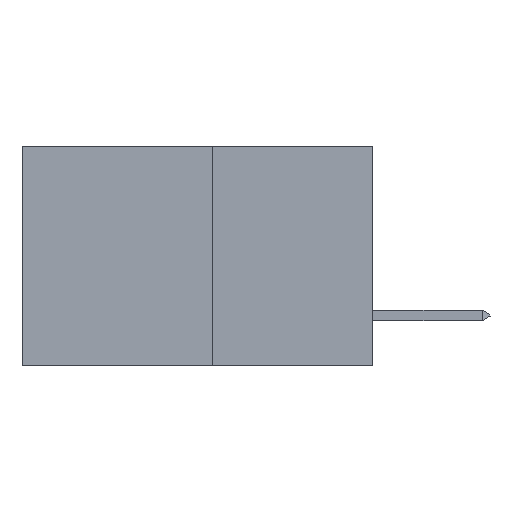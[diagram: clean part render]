
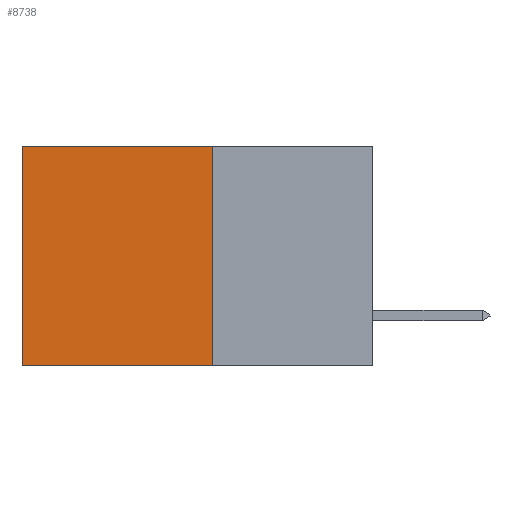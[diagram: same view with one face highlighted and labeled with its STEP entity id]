
A CAD part, left-side view. The second image highlights one B-rep face of the part: STEP entity #8738.
In plain terms, the highlighted planar face has unit normal (-1, 0, 0).
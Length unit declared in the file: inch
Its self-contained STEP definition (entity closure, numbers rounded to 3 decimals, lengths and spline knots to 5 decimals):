
#4 = CARTESIAN_POINT ( 'NONE',  ( 0.277, 0.27, -0.37 ) ) ;
#150 = CARTESIAN_POINT ( 'NONE',  ( 0.277, 0.59, 0. ) ) ;
#162 = EDGE_LOOP ( 'NONE', ( #10276, #10922, #11803, #12343 ) ) ;
#548 = EDGE_CURVE ( 'NONE', #7776, #759, #12877, .T. ) ;
#759 = VERTEX_POINT ( 'NONE', #3535 ) ;
#1396 = VECTOR ( 'NONE', #1722, 39.37008 ) ;
#1722 = DIRECTION ( 'NONE',  ( 0., 0., -1. ) ) ;
#1736 = CARTESIAN_POINT ( 'NONE',  ( 0.277, 0.27, -0.37 ) ) ;
#2013 = EDGE_CURVE ( 'NONE', #13801, #759, #10523, .T. ) ;
#2250 = PLANE ( 'NONE',  #7440 ) ;
#2953 = LINE ( 'NONE', #6806, #5700 ) ;
#3085 = VERTEX_POINT ( 'NONE', #13386 ) ;
#3471 = DIRECTION ( 'NONE',  ( 1., 0., 0. ) ) ;
#3535 = CARTESIAN_POINT ( 'NONE',  ( 0.277, 0.59, -0.37 ) ) ;
#5170 = EDGE_CURVE ( 'NONE', #3085, #7776, #9796, .T. ) ;
#5700 = VECTOR ( 'NONE', #14391, 39.37008 ) ;
#6550 = DIRECTION ( 'NONE',  ( 0., 0., -1. ) ) ;
#6665 = CARTESIAN_POINT ( 'NONE',  ( 0.277, 0.59, -0.37 ) ) ;
#6806 = CARTESIAN_POINT ( 'NONE',  ( 0.277, 0.27, 0. ) ) ;
#6930 = FACE_OUTER_BOUND ( 'NONE', #162, .T. ) ;
#7097 = VECTOR ( 'NONE', #7107, 39.37008 ) ;
#7107 = DIRECTION ( 'NONE',  ( 0., 1., 0. ) ) ;
#7440 = AXIS2_PLACEMENT_3D ( 'NONE', #4, #3471, #11352 ) ;
#7587 = VECTOR ( 'NONE', #6550, 39.37008 ) ;
#7776 = VERTEX_POINT ( 'NONE', #8475 ) ;
#8475 = CARTESIAN_POINT ( 'NONE',  ( 0.277, 0.27, -0.37 ) ) ;
#8738 = ADVANCED_FACE ( 'NONE', ( #6930 ), #2250, .F. ) ;
#9796 = LINE ( 'NONE', #1736, #1396 ) ;
#10276 = ORIENTED_EDGE ( 'NONE', *, *, #2013, .T. ) ;
#10446 = CARTESIAN_POINT ( 'NONE',  ( 0.277, 0.27, -0.37 ) ) ;
#10523 = LINE ( 'NONE', #6665, #7587 ) ;
#10922 = ORIENTED_EDGE ( 'NONE', *, *, #548, .F. ) ;
#11352 = DIRECTION ( 'NONE',  ( 0., 0., -1. ) ) ;
#11803 = ORIENTED_EDGE ( 'NONE', *, *, #5170, .F. ) ;
#12343 = ORIENTED_EDGE ( 'NONE', *, *, #13662, .T. ) ;
#12877 = LINE ( 'NONE', #10446, #7097 ) ;
#13386 = CARTESIAN_POINT ( 'NONE',  ( 0.277, 0.27, 0. ) ) ;
#13662 = EDGE_CURVE ( 'NONE', #3085, #13801, #2953, .T. ) ;
#13801 = VERTEX_POINT ( 'NONE', #150 ) ;
#14391 = DIRECTION ( 'NONE',  ( 0., 1., 0. ) ) ;
